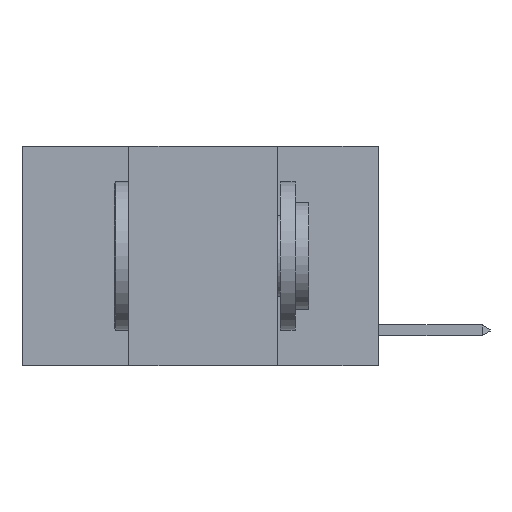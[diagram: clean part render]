
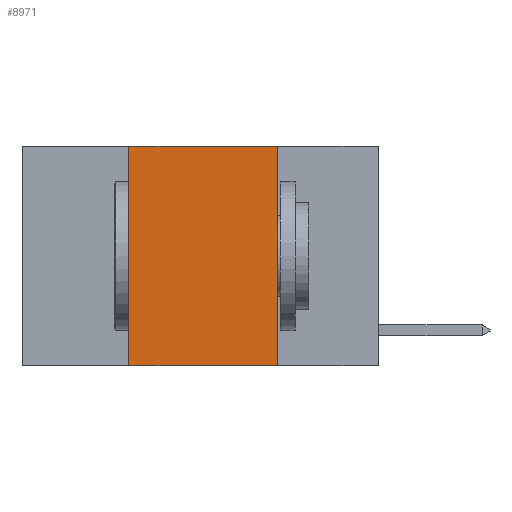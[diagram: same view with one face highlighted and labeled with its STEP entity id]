
A CAD part, left-side view. The second image highlights one B-rep face of the part: STEP entity #8971.
In plain terms, the highlighted planar face has unit normal (-1, 0, 0).
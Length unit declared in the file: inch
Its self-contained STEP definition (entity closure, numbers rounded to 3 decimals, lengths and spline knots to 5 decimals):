
#728 = LINE ( 'NONE', #7585, #2854 ) ;
#1007 = VERTEX_POINT ( 'NONE', #7854 ) ;
#1516 = CARTESIAN_POINT ( 'NONE',  ( 0., 0.17, 0. ) ) ;
#1572 = FACE_OUTER_BOUND ( 'NONE', #2979, .T. ) ;
#2217 = AXIS2_PLACEMENT_3D ( 'NONE', #7555, #8429, #3241 ) ;
#2322 = PLANE ( 'NONE',  #2217 ) ;
#2459 = DIRECTION ( 'NONE',  ( 0., 0., -1. ) ) ;
#2473 = LINE ( 'NONE', #3262, #6840 ) ;
#2854 = VECTOR ( 'NONE', #5861, 39.37008 ) ;
#2979 = EDGE_LOOP ( 'NONE', ( #5211, #7484, #5740, #10362 ) ) ;
#3053 = VECTOR ( 'NONE', #2459, 39.37008 ) ;
#3241 = DIRECTION ( 'NONE',  ( 0., 0., -1. ) ) ;
#3262 = CARTESIAN_POINT ( 'NONE',  ( 0., 0.6, 0. ) ) ;
#3329 = DIRECTION ( 'NONE',  ( 0., 0., 1. ) ) ;
#3715 = VECTOR ( 'NONE', #3329, 39.37008 ) ;
#4091 = VERTEX_POINT ( 'NONE', #5878 ) ;
#4276 = CARTESIAN_POINT ( 'NONE',  ( 0., 0.17, 0. ) ) ;
#4783 = VERTEX_POINT ( 'NONE', #7883 ) ;
#5032 = DIRECTION ( 'NONE',  ( 0., -1., 0. ) ) ;
#5211 = ORIENTED_EDGE ( 'NONE', *, *, #7094, .F. ) ;
#5740 = ORIENTED_EDGE ( 'NONE', *, *, #11254, .F. ) ;
#5861 = DIRECTION ( 'NONE',  ( 0., -1., 0. ) ) ;
#5878 = CARTESIAN_POINT ( 'NONE',  ( 0., 0.17, -0.37 ) ) ;
#5913 = CARTESIAN_POINT ( 'NONE',  ( 0., 0.42, 0. ) ) ;
#5946 = VERTEX_POINT ( 'NONE', #4276 ) ;
#6267 = LINE ( 'NONE', #5913, #3715 ) ;
#6840 = VECTOR ( 'NONE', #5032, 39.37008 ) ;
#7094 = EDGE_CURVE ( 'NONE', #5946, #4091, #7674, .T. ) ;
#7484 = ORIENTED_EDGE ( 'NONE', *, *, #10742, .F. ) ;
#7555 = CARTESIAN_POINT ( 'NONE',  ( 0., 0.6, 0. ) ) ;
#7585 = CARTESIAN_POINT ( 'NONE',  ( 0., 0.6, -0.37 ) ) ;
#7674 = LINE ( 'NONE', #1516, #3053 ) ;
#7854 = CARTESIAN_POINT ( 'NONE',  ( 0., 0.42, -0.37 ) ) ;
#7883 = CARTESIAN_POINT ( 'NONE',  ( 0., 0.42, 0. ) ) ;
#8429 = DIRECTION ( 'NONE',  ( 1., 0., 0. ) ) ;
#8971 = ADVANCED_FACE ( 'NONE', ( #1572 ), #2322, .F. ) ;
#9508 = EDGE_CURVE ( 'NONE', #1007, #4091, #728, .T. ) ;
#10362 = ORIENTED_EDGE ( 'NONE', *, *, #9508, .T. ) ;
#10742 = EDGE_CURVE ( 'NONE', #4783, #5946, #2473, .T. ) ;
#11254 = EDGE_CURVE ( 'NONE', #1007, #4783, #6267, .T. ) ;
